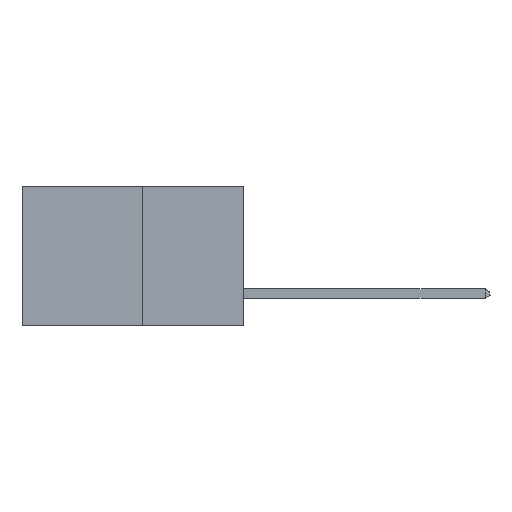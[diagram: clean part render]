
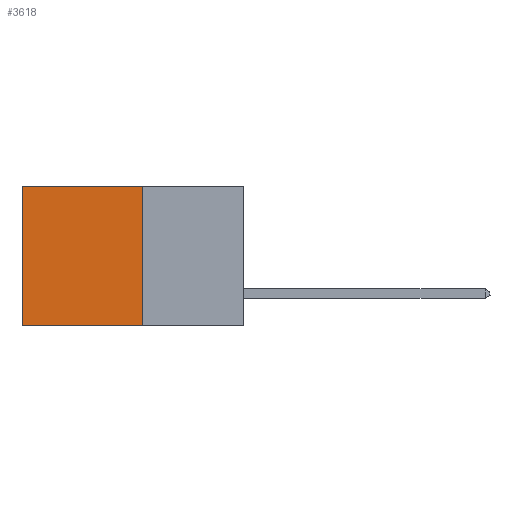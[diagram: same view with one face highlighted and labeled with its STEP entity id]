
A CAD part, left-side view. The second image highlights one B-rep face of the part: STEP entity #3618.
In plain terms, the highlighted planar face has unit normal (-1, 0, 0).
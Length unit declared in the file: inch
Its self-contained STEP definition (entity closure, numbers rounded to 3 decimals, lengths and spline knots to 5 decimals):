
#624 = FACE_OUTER_BOUND ( 'NONE', #1010, .T. ) ;
#1010 = EDGE_LOOP ( 'NONE', ( #6351, #5820, #4709, #5231 ) ) ;
#1029 = CARTESIAN_POINT ( 'NONE',  ( 0.277, 0.27, -0.37 ) ) ;
#1054 = LINE ( 'NONE', #2584, #6744 ) ;
#1292 = LINE ( 'NONE', #1487, #8423 ) ;
#1398 = VERTEX_POINT ( 'NONE', #3580 ) ;
#1487 = CARTESIAN_POINT ( 'NONE',  ( 0.277, 0.59, -0.37 ) ) ;
#1498 = EDGE_CURVE ( 'NONE', #7098, #3699, #7177, .T. ) ;
#1969 = DIRECTION ( 'NONE',  ( 0., 0., -1. ) ) ;
#1983 = DIRECTION ( 'NONE',  ( 1., 0., 0. ) ) ;
#1992 = PLANE ( 'NONE',  #5030 ) ;
#2042 = EDGE_CURVE ( 'NONE', #1398, #8254, #1054, .T. ) ;
#2568 = DIRECTION ( 'NONE',  ( 0., 1., 0. ) ) ;
#2584 = CARTESIAN_POINT ( 'NONE',  ( 0.277, 0.27, 0. ) ) ;
#3580 = CARTESIAN_POINT ( 'NONE',  ( 0.277, 0.27, 0. ) ) ;
#3618 = ADVANCED_FACE ( 'NONE', ( #624 ), #1992, .F. ) ;
#3699 = VERTEX_POINT ( 'NONE', #7595 ) ;
#3734 = EDGE_CURVE ( 'NONE', #8254, #3699, #1292, .T. ) ;
#4007 = DIRECTION ( 'NONE',  ( 0., 0., -1. ) ) ;
#4615 = EDGE_CURVE ( 'NONE', #1398, #7098, #7417, .T. ) ;
#4709 = ORIENTED_EDGE ( 'NONE', *, *, #4615, .F. ) ;
#4957 = CARTESIAN_POINT ( 'NONE',  ( 0.277, 0.59, 0. ) ) ;
#5030 = AXIS2_PLACEMENT_3D ( 'NONE', #8686, #1983, #1969 ) ;
#5231 = ORIENTED_EDGE ( 'NONE', *, *, #2042, .T. ) ;
#5413 = VECTOR ( 'NONE', #7942, 39.37008 ) ;
#5820 = ORIENTED_EDGE ( 'NONE', *, *, #1498, .F. ) ;
#6315 = DIRECTION ( 'NONE',  ( 0., 1., 0. ) ) ;
#6351 = ORIENTED_EDGE ( 'NONE', *, *, #3734, .T. ) ;
#6398 = CARTESIAN_POINT ( 'NONE',  ( 0.277, 0.27, -0.37 ) ) ;
#6744 = VECTOR ( 'NONE', #2568, 39.37008 ) ;
#6968 = VECTOR ( 'NONE', #6315, 39.37008 ) ;
#7098 = VERTEX_POINT ( 'NONE', #1029 ) ;
#7177 = LINE ( 'NONE', #6398, #6968 ) ;
#7417 = LINE ( 'NONE', #8133, #5413 ) ;
#7595 = CARTESIAN_POINT ( 'NONE',  ( 0.277, 0.59, -0.37 ) ) ;
#7942 = DIRECTION ( 'NONE',  ( 0., 0., -1. ) ) ;
#8133 = CARTESIAN_POINT ( 'NONE',  ( 0.277, 0.27, -0.37 ) ) ;
#8254 = VERTEX_POINT ( 'NONE', #4957 ) ;
#8423 = VECTOR ( 'NONE', #4007, 39.37008 ) ;
#8686 = CARTESIAN_POINT ( 'NONE',  ( 0.277, 0.27, -0.37 ) ) ;
